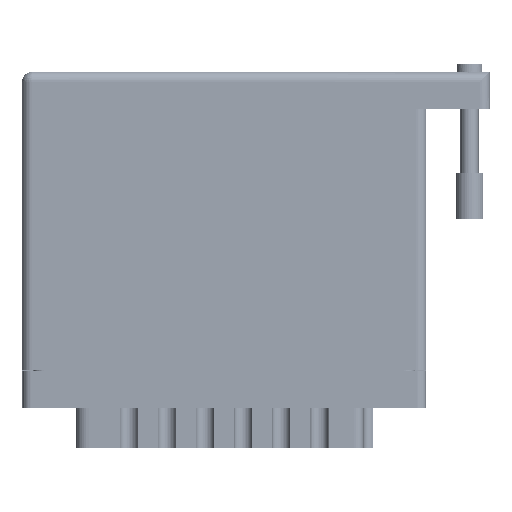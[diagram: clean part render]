
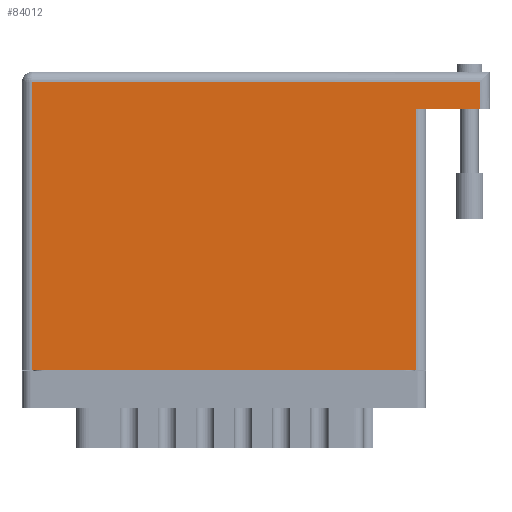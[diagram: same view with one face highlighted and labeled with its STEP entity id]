
A CAD part, front view. The second image highlights one B-rep face of the part: STEP entity #84012.
In plain terms, the highlighted face is planar.
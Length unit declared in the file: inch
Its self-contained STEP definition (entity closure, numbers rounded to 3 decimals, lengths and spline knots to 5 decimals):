
#1987 = CARTESIAN_POINT ( 'NONE',  ( 0.07, 0., 0. ) ) ;
#2938 = DIRECTION ( 'NONE',  ( 0., -1., 0. ) ) ;
#6803 = ORIENTED_EDGE ( 'NONE', *, *, #85858, .T. ) ;
#8757 = VERTEX_POINT ( 'NONE', #59738 ) ;
#9374 = VECTOR ( 'NONE', #2938, 39.37008 ) ;
#13644 = VERTEX_POINT ( 'NONE', #83061 ) ;
#17851 = EDGE_CURVE ( 'NONE', #13644, #33289, #53821, .T. ) ;
#18733 = ORIENTED_EDGE ( 'NONE', *, *, #72575, .F. ) ;
#20743 = VECTOR ( 'NONE', #28062, 39.37008 ) ;
#22124 = VECTOR ( 'NONE', #96416, 39.37008 ) ;
#24734 = VECTOR ( 'NONE', #80740, 39.37008 ) ;
#26971 = LINE ( 'NONE', #45267, #74689 ) ;
#27665 = CARTESIAN_POINT ( 'NONE',  ( 0., 2.03, 0. ) ) ;
#28062 = DIRECTION ( 'NONE',  ( 1., 0., 0. ) ) ;
#33289 = VERTEX_POINT ( 'NONE', #82138 ) ;
#33934 = LINE ( 'NONE', #95450, #85139 ) ;
#34066 = VERTEX_POINT ( 'NONE', #56523 ) ;
#35103 = EDGE_CURVE ( 'NONE', #34066, #8757, #66411, .T. ) ;
#36870 = CARTESIAN_POINT ( 'NONE',  ( 3.12, 2.03, 0. ) ) ;
#38440 = EDGE_LOOP ( 'NONE', ( #6803, #68461, #18733, #57974, #63199, #68723 ) ) ;
#41209 = VERTEX_POINT ( 'NONE', #65148 ) ;
#42421 = CARTESIAN_POINT ( 'NONE',  ( 0.07, 1.96, 0. ) ) ;
#42730 = DIRECTION ( 'NONE',  ( -1., 0., 0. ) ) ;
#45267 = CARTESIAN_POINT ( 'NONE',  ( 3.19, 1.774, 0. ) ) ;
#48769 = LINE ( 'NONE', #95809, #20743 ) ;
#53821 = LINE ( 'NONE', #73272, #24734 ) ;
#56523 = CARTESIAN_POINT ( 'NONE',  ( 3.12, 1.774, 0. ) ) ;
#57974 = ORIENTED_EDGE ( 'NONE', *, *, #35103, .T. ) ;
#58310 = PLANE ( 'NONE',  #64772 ) ;
#59738 = CARTESIAN_POINT ( 'NONE',  ( 3.12, 1.96, 0. ) ) ;
#61931 = FACE_OUTER_BOUND ( 'NONE', #38440, .T. ) ;
#63199 = ORIENTED_EDGE ( 'NONE', *, *, #72953, .T. ) ;
#64772 = AXIS2_PLACEMENT_3D ( 'NONE', #27665, #71938, #42730 ) ;
#65148 = CARTESIAN_POINT ( 'NONE',  ( 0.07, 0., 0. ) ) ;
#66411 = LINE ( 'NONE', #36870, #22124 ) ;
#68461 = ORIENTED_EDGE ( 'NONE', *, *, #17851, .T. ) ;
#68723 = ORIENTED_EDGE ( 'NONE', *, *, #91556, .T. ) ;
#71938 = DIRECTION ( 'NONE',  ( 0., 0., -1. ) ) ;
#72575 = EDGE_CURVE ( 'NONE', #34066, #33289, #26971, .T. ) ;
#72953 = EDGE_CURVE ( 'NONE', #8757, #94818, #33934, .T. ) ;
#73265 = DIRECTION ( 'NONE',  ( -1., 0., 0. ) ) ;
#73272 = CARTESIAN_POINT ( 'NONE',  ( 2.685, 1.774, 0. ) ) ;
#74689 = VECTOR ( 'NONE', #91765, 39.37008 ) ;
#80740 = DIRECTION ( 'NONE',  ( 0., 1., 0. ) ) ;
#82138 = CARTESIAN_POINT ( 'NONE',  ( 2.685, 1.774, 0. ) ) ;
#83061 = CARTESIAN_POINT ( 'NONE',  ( 2.685, 0., 0. ) ) ;
#84012 = ADVANCED_FACE ( 'NONE', ( #61931 ), #58310, .F. ) ;
#85139 = VECTOR ( 'NONE', #73265, 39.37008 ) ;
#85858 = EDGE_CURVE ( 'NONE', #41209, #13644, #48769, .T. ) ;
#91556 = EDGE_CURVE ( 'NONE', #94818, #41209, #93291, .T. ) ;
#91765 = DIRECTION ( 'NONE',  ( -1., 0., 0. ) ) ;
#93291 = LINE ( 'NONE', #1987, #9374 ) ;
#94818 = VERTEX_POINT ( 'NONE', #42421 ) ;
#95450 = CARTESIAN_POINT ( 'NONE',  ( 0., 1.96, 0. ) ) ;
#95809 = CARTESIAN_POINT ( 'NONE',  ( 0., 0., 0. ) ) ;
#96416 = DIRECTION ( 'NONE',  ( 0., 1., 0. ) ) ;
